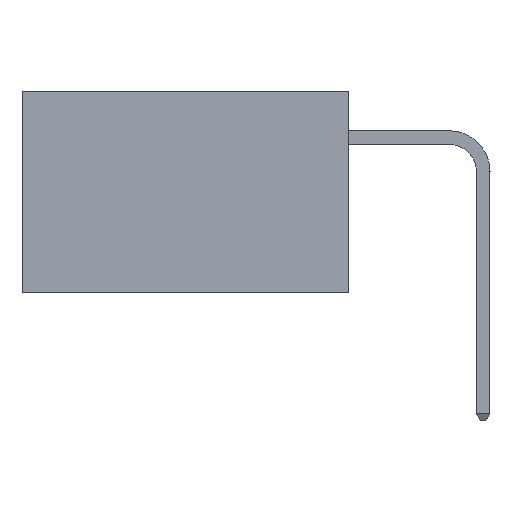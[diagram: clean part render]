
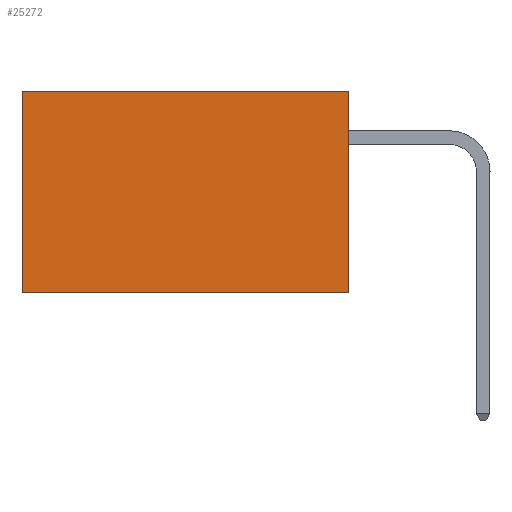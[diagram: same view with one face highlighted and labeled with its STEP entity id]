
A CAD part, left-side view. The second image highlights one B-rep face of the part: STEP entity #25272.
In plain terms, the highlighted planar face has unit normal (-1, 0, 0).
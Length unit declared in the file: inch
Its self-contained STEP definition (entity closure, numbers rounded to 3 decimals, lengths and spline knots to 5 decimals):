
#1369 = PLANE ( 'NONE',  #24795 ) ;
#2301 = EDGE_LOOP ( 'NONE', ( #46737, #30071, #21888, #23993 ) ) ;
#4274 = FACE_OUTER_BOUND ( 'NONE', #2301, .T. ) ;
#4367 = VECTOR ( 'NONE', #40597, 39.37008 ) ;
#5091 = VERTEX_POINT ( 'NONE', #42534 ) ;
#5108 = DIRECTION ( 'NONE',  ( 1., 0., 0. ) ) ;
#5414 = EDGE_CURVE ( 'NONE', #14010, #15590, #23921, .T. ) ;
#9173 = DIRECTION ( 'NONE',  ( 0., 1., 0. ) ) ;
#14010 = VERTEX_POINT ( 'NONE', #20691 ) ;
#15590 = VERTEX_POINT ( 'NONE', #21922 ) ;
#16211 = LINE ( 'NONE', #27443, #35652 ) ;
#20691 = CARTESIAN_POINT ( 'NONE',  ( 0.2875, 0., -0.37 ) ) ;
#21165 = LINE ( 'NONE', #33272, #39454 ) ;
#21888 = ORIENTED_EDGE ( 'NONE', *, *, #42088, .F. ) ;
#21922 = CARTESIAN_POINT ( 'NONE',  ( 0.2875, 0.6, -0.37 ) ) ;
#23487 = VECTOR ( 'NONE', #32849, 39.37008 ) ;
#23921 = LINE ( 'NONE', #36933, #4367 ) ;
#23993 = ORIENTED_EDGE ( 'NONE', *, *, #46195, .T. ) ;
#24363 = VERTEX_POINT ( 'NONE', #40408 ) ;
#24795 = AXIS2_PLACEMENT_3D ( 'NONE', #34265, #5108, #30725 ) ;
#25272 = ADVANCED_FACE ( 'NONE', ( #4274 ), #1369, .F. ) ;
#27443 = CARTESIAN_POINT ( 'NONE',  ( 0.2875, 0., 0. ) ) ;
#30071 = ORIENTED_EDGE ( 'NONE', *, *, #5414, .F. ) ;
#30725 = DIRECTION ( 'NONE',  ( 0., 0., -1. ) ) ;
#32849 = DIRECTION ( 'NONE',  ( 0., 0., -1. ) ) ;
#33272 = CARTESIAN_POINT ( 'NONE',  ( 0.2875, 0.6, 0. ) ) ;
#34265 = CARTESIAN_POINT ( 'NONE',  ( 0.2875, 0., 0. ) ) ;
#35652 = VECTOR ( 'NONE', #9173, 39.37008 ) ;
#36933 = CARTESIAN_POINT ( 'NONE',  ( 0.2875, 0., -0.37 ) ) ;
#39454 = VECTOR ( 'NONE', #44137, 39.37008 ) ;
#40408 = CARTESIAN_POINT ( 'NONE',  ( 0.2875, 0., 0. ) ) ;
#40597 = DIRECTION ( 'NONE',  ( 0., 1., 0. ) ) ;
#42088 = EDGE_CURVE ( 'NONE', #24363, #14010, #44023, .T. ) ;
#42534 = CARTESIAN_POINT ( 'NONE',  ( 0.2875, 0.6, 0. ) ) ;
#42841 = EDGE_CURVE ( 'NONE', #5091, #15590, #21165, .T. ) ;
#44023 = LINE ( 'NONE', #47362, #23487 ) ;
#44137 = DIRECTION ( 'NONE',  ( 0., 0., -1. ) ) ;
#46195 = EDGE_CURVE ( 'NONE', #24363, #5091, #16211, .T. ) ;
#46737 = ORIENTED_EDGE ( 'NONE', *, *, #42841, .T. ) ;
#47362 = CARTESIAN_POINT ( 'NONE',  ( 0.2875, 0., 0. ) ) ;
